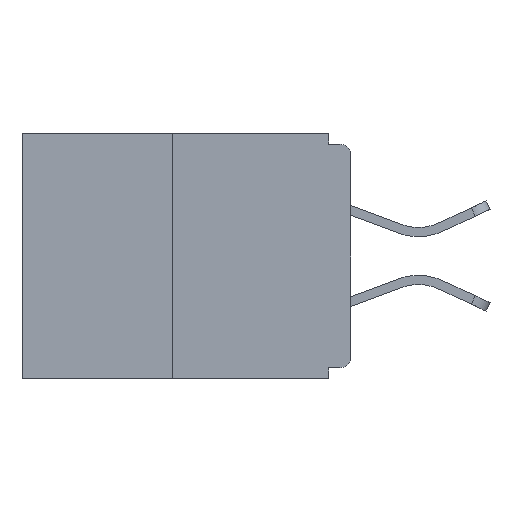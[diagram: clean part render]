
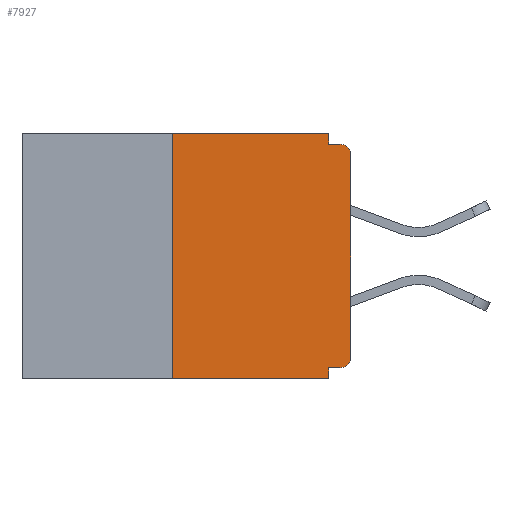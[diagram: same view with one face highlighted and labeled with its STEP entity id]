
A CAD part, left-side view. The second image highlights one B-rep face of the part: STEP entity #7927.
In plain terms, the highlighted planar face has unit normal (-1, 0, 0).
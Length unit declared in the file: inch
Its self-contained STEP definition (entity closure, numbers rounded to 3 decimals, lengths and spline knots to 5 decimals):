
#473 = CARTESIAN_POINT ( 'NONE',  ( 0., 0.031, 0. ) ) ;
#769 = CARTESIAN_POINT ( 'NONE',  ( 0., 0., -0.015 ) ) ;
#2272 = VERTEX_POINT ( 'NONE', #23836 ) ;
#2305 = CARTESIAN_POINT ( 'NONE',  ( 0., 0.015, -0.03 ) ) ;
#2328 = LINE ( 'NONE', #9152, #4342 ) ;
#2427 = CARTESIAN_POINT ( 'NONE',  ( 0., 0., 0. ) ) ;
#2517 = AXIS2_PLACEMENT_3D ( 'NONE', #17255, #19128, #11858 ) ;
#2563 = VECTOR ( 'NONE', #16693, 39.37008 ) ;
#2573 = EDGE_CURVE ( 'NONE', #10931, #17592, #9676, .T. ) ;
#2867 = PLANE ( 'NONE',  #7727 ) ;
#2962 = CARTESIAN_POINT ( 'NONE',  ( 0., 0.46, 0. ) ) ;
#3704 = VERTEX_POINT ( 'NONE', #3899 ) ;
#3899 = CARTESIAN_POINT ( 'NONE',  ( 0., 0.015, -0.015 ) ) ;
#4114 = LINE ( 'NONE', #769, #20158 ) ;
#4301 = VERTEX_POINT ( 'NONE', #17021 ) ;
#4307 = LINE ( 'NONE', #16384, #2563 ) ;
#4342 = VECTOR ( 'NONE', #10982, 39.37008 ) ;
#4468 = VERTEX_POINT ( 'NONE', #13690 ) ;
#4498 = ORIENTED_EDGE ( 'NONE', *, *, #2573, .F. ) ;
#4710 = ORIENTED_EDGE ( 'NONE', *, *, #21569, .F. ) ;
#5196 = DIRECTION ( 'NONE',  ( 0., 0., 1. ) ) ;
#5810 = ORIENTED_EDGE ( 'NONE', *, *, #10800, .F. ) ;
#5946 = VECTOR ( 'NONE', #5196, 39.37008 ) ;
#6010 = ORIENTED_EDGE ( 'NONE', *, *, #9438, .T. ) ;
#6025 = CIRCLE ( 'NONE', #19221, 0.015 ) ;
#6262 = DIRECTION ( 'NONE',  ( 1., 0., 0. ) ) ;
#6494 = CARTESIAN_POINT ( 'NONE',  ( 0., 0.46, 0. ) ) ;
#6635 = CARTESIAN_POINT ( 'NONE',  ( 0., 0.031, 0. ) ) ;
#6671 = FACE_OUTER_BOUND ( 'NONE', #19830, .T. ) ;
#7339 = ORIENTED_EDGE ( 'NONE', *, *, #23247, .T. ) ;
#7727 = AXIS2_PLACEMENT_3D ( 'NONE', #6494, #6262, #22819 ) ;
#7927 = ADVANCED_FACE ( 'NONE', ( #6671 ), #2867, .F. ) ;
#8015 = VERTEX_POINT ( 'NONE', #10480 ) ;
#8269 = DIRECTION ( 'NONE',  ( 0., 0., 1. ) ) ;
#9152 = CARTESIAN_POINT ( 'NONE',  ( 0., 0., -0.328 ) ) ;
#9295 = EDGE_CURVE ( 'NONE', #4301, #22671, #15796, .T. ) ;
#9438 = EDGE_CURVE ( 'NONE', #4468, #4301, #10322, .T. ) ;
#9676 = LINE ( 'NONE', #11874, #5946 ) ;
#9735 = ORIENTED_EDGE ( 'NONE', *, *, #21682, .F. ) ;
#9920 = DIRECTION ( 'NONE',  ( 0., -1., 0. ) ) ;
#10286 = LINE ( 'NONE', #6635, #19186 ) ;
#10322 = CIRCLE ( 'NONE', #2517, 0.015 ) ;
#10441 = CARTESIAN_POINT ( 'NONE',  ( 0., 0.031, -0.343 ) ) ;
#10480 = CARTESIAN_POINT ( 'NONE',  ( 0., 0.031, -0.343 ) ) ;
#10800 = EDGE_CURVE ( 'NONE', #11359, #2272, #10286, .T. ) ;
#10931 = VERTEX_POINT ( 'NONE', #18381 ) ;
#10982 = DIRECTION ( 'NONE',  ( 0., 1., 0. ) ) ;
#11359 = VERTEX_POINT ( 'NONE', #473 ) ;
#11543 = ORIENTED_EDGE ( 'NONE', *, *, #9295, .T. ) ;
#11656 = EDGE_CURVE ( 'NONE', #13465, #8015, #15447, .T. ) ;
#11858 = DIRECTION ( 'NONE',  ( 0., 0., -1. ) ) ;
#11874 = CARTESIAN_POINT ( 'NONE',  ( 0., 0.25, 0. ) ) ;
#11909 = DIRECTION ( 'NONE',  ( 0., -1., 0. ) ) ;
#12051 = ORIENTED_EDGE ( 'NONE', *, *, #11656, .F. ) ;
#12257 = VECTOR ( 'NONE', #18051, 39.37008 ) ;
#12747 = CARTESIAN_POINT ( 'NONE',  ( 0., 0.031, -0.328 ) ) ;
#13465 = VERTEX_POINT ( 'NONE', #12747 ) ;
#13690 = CARTESIAN_POINT ( 'NONE',  ( 0., 0.015, -0.328 ) ) ;
#14642 = CARTESIAN_POINT ( 'NONE',  ( 0., 0., -0.03 ) ) ;
#15183 = DIRECTION ( 'NONE',  ( -1., 0., 0. ) ) ;
#15447 = LINE ( 'NONE', #10441, #12257 ) ;
#15796 = LINE ( 'NONE', #2427, #19218 ) ;
#16107 = ORIENTED_EDGE ( 'NONE', *, *, #22888, .F. ) ;
#16290 = CARTESIAN_POINT ( 'NONE',  ( 0., 0.25, 0. ) ) ;
#16384 = CARTESIAN_POINT ( 'NONE',  ( 0., 0.46, -0.343 ) ) ;
#16693 = DIRECTION ( 'NONE',  ( 0., -1., 0. ) ) ;
#16837 = ORIENTED_EDGE ( 'NONE', *, *, #18699, .T. ) ;
#17021 = CARTESIAN_POINT ( 'NONE',  ( 0., 0., -0.313 ) ) ;
#17255 = CARTESIAN_POINT ( 'NONE',  ( 0., 0.015, -0.313 ) ) ;
#17592 = VERTEX_POINT ( 'NONE', #16290 ) ;
#17652 = DIRECTION ( 'NONE',  ( 0., 0., -1. ) ) ;
#18051 = DIRECTION ( 'NONE',  ( 0., 0., -1. ) ) ;
#18381 = CARTESIAN_POINT ( 'NONE',  ( 0., 0.25, -0.343 ) ) ;
#18699 = EDGE_CURVE ( 'NONE', #10931, #8015, #4307, .T. ) ;
#19128 = DIRECTION ( 'NONE',  ( -1., 0., 0. ) ) ;
#19186 = VECTOR ( 'NONE', #17652, 39.37008 ) ;
#19218 = VECTOR ( 'NONE', #8269, 39.37008 ) ;
#19221 = AXIS2_PLACEMENT_3D ( 'NONE', #2305, #15183, #22724 ) ;
#19830 = EDGE_LOOP ( 'NONE', ( #4710, #4498, #16837, #12051, #16107, #6010, #11543, #7339, #9735, #5810 ) ) ;
#20158 = VECTOR ( 'NONE', #9920, 39.37008 ) ;
#21569 = EDGE_CURVE ( 'NONE', #17592, #11359, #23335, .T. ) ;
#21682 = EDGE_CURVE ( 'NONE', #2272, #3704, #4114, .T. ) ;
#22671 = VERTEX_POINT ( 'NONE', #14642 ) ;
#22724 = DIRECTION ( 'NONE',  ( 0., 0., -1. ) ) ;
#22819 = DIRECTION ( 'NONE',  ( 0., 0., -1. ) ) ;
#22888 = EDGE_CURVE ( 'NONE', #4468, #13465, #2328, .T. ) ;
#23247 = EDGE_CURVE ( 'NONE', #22671, #3704, #6025, .T. ) ;
#23335 = LINE ( 'NONE', #2962, #23648 ) ;
#23648 = VECTOR ( 'NONE', #11909, 39.37008 ) ;
#23836 = CARTESIAN_POINT ( 'NONE',  ( 0., 0.031, -0.015 ) ) ;
